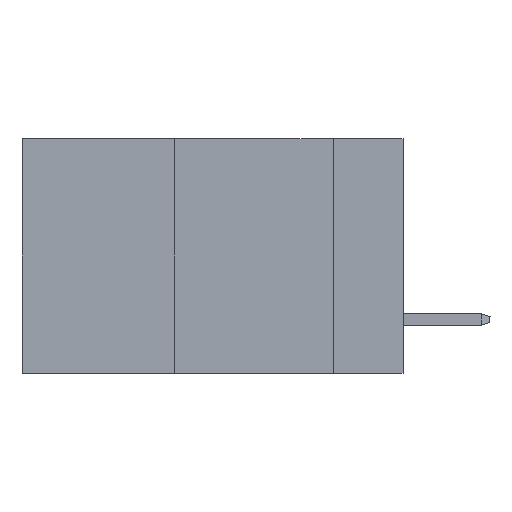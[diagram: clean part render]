
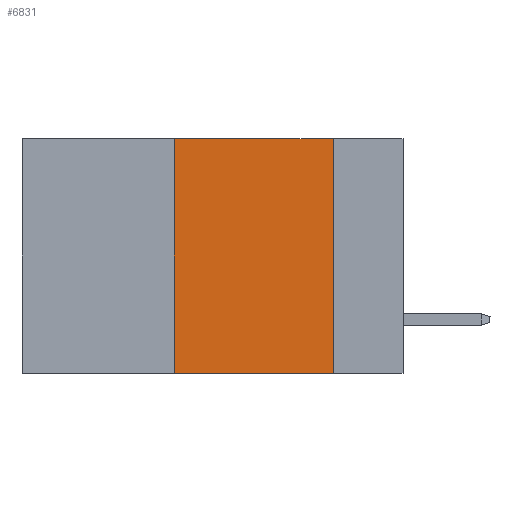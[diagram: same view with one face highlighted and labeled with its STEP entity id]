
A CAD part, left-side view. The second image highlights one B-rep face of the part: STEP entity #6831.
In plain terms, the highlighted planar face has unit normal (-1, 0, 0).
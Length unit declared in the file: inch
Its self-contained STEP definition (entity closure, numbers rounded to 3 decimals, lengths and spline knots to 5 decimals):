
#551 = LINE ( 'NONE', #2261, #12378 ) ;
#608 = CARTESIAN_POINT ( 'NONE',  ( 0., 0.11, 0. ) ) ;
#1107 = ORIENTED_EDGE ( 'NONE', *, *, #2838, .F. ) ;
#1554 = DIRECTION ( 'NONE',  ( 0., -1., 0. ) ) ;
#1627 = CARTESIAN_POINT ( 'NONE',  ( 0., 0.6, 0. ) ) ;
#1825 = ORIENTED_EDGE ( 'NONE', *, *, #11745, .F. ) ;
#2261 = CARTESIAN_POINT ( 'NONE',  ( 0., 0.6, -0.37 ) ) ;
#2582 = VERTEX_POINT ( 'NONE', #3823 ) ;
#2718 = DIRECTION ( 'NONE',  ( 0., 0., -1. ) ) ;
#2838 = EDGE_CURVE ( 'NONE', #2582, #5793, #9172, .T. ) ;
#2991 = ORIENTED_EDGE ( 'NONE', *, *, #10001, .T. ) ;
#3294 = DIRECTION ( 'NONE',  ( 0., 0., -1. ) ) ;
#3823 = CARTESIAN_POINT ( 'NONE',  ( 0., 0.36, -0.37 ) ) ;
#4644 = FACE_OUTER_BOUND ( 'NONE', #11299, .T. ) ;
#5010 = VECTOR ( 'NONE', #1554, 39.37008 ) ;
#5546 = CARTESIAN_POINT ( 'NONE',  ( 0., 0.11, -0.37 ) ) ;
#5725 = PLANE ( 'NONE',  #6441 ) ;
#5793 = VERTEX_POINT ( 'NONE', #9216 ) ;
#6227 = LINE ( 'NONE', #7122, #5010 ) ;
#6441 = AXIS2_PLACEMENT_3D ( 'NONE', #1627, #6689, #2718 ) ;
#6689 = DIRECTION ( 'NONE',  ( 1., 0., 0. ) ) ;
#6831 = ADVANCED_FACE ( 'NONE', ( #4644 ), #5725, .F. ) ;
#7122 = CARTESIAN_POINT ( 'NONE',  ( 0., 0.6, 0. ) ) ;
#7260 = CARTESIAN_POINT ( 'NONE',  ( 0., 0.36, 0. ) ) ;
#8349 = DIRECTION ( 'NONE',  ( 0., -1., 0. ) ) ;
#9115 = DIRECTION ( 'NONE',  ( 0., 0., 1. ) ) ;
#9172 = LINE ( 'NONE', #7260, #11480 ) ;
#9216 = CARTESIAN_POINT ( 'NONE',  ( 0., 0.36, 0. ) ) ;
#9561 = EDGE_CURVE ( 'NONE', #9929, #11477, #10313, .T. ) ;
#9929 = VERTEX_POINT ( 'NONE', #10890 ) ;
#10001 = EDGE_CURVE ( 'NONE', #2582, #11477, #551, .T. ) ;
#10047 = ORIENTED_EDGE ( 'NONE', *, *, #9561, .F. ) ;
#10152 = VECTOR ( 'NONE', #3294, 39.37008 ) ;
#10313 = LINE ( 'NONE', #608, #10152 ) ;
#10890 = CARTESIAN_POINT ( 'NONE',  ( 0., 0.11, 0. ) ) ;
#11299 = EDGE_LOOP ( 'NONE', ( #10047, #1825, #1107, #2991 ) ) ;
#11477 = VERTEX_POINT ( 'NONE', #5546 ) ;
#11480 = VECTOR ( 'NONE', #9115, 39.37008 ) ;
#11745 = EDGE_CURVE ( 'NONE', #5793, #9929, #6227, .T. ) ;
#12378 = VECTOR ( 'NONE', #8349, 39.37008 ) ;
